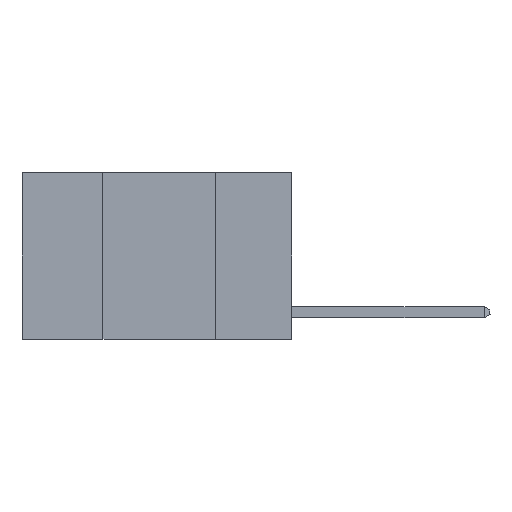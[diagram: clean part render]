
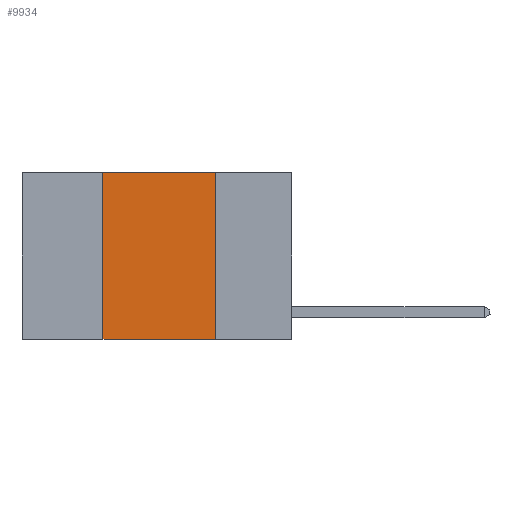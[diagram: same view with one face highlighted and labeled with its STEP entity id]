
A CAD part, left-side view. The second image highlights one B-rep face of the part: STEP entity #9934.
In plain terms, the highlighted planar face has unit normal (-1, 0, 0).
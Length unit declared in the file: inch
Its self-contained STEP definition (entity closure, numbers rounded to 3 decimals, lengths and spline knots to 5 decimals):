
#4 = VERTEX_POINT ( 'NONE', #1848 ) ;
#546 = CARTESIAN_POINT ( 'NONE',  ( 0., 0.6, 0. ) ) ;
#758 = PLANE ( 'NONE',  #8987 ) ;
#1290 = DIRECTION ( 'NONE',  ( 0., -1., 0. ) ) ;
#1499 = DIRECTION ( 'NONE',  ( 0., 0., -1. ) ) ;
#1561 = CARTESIAN_POINT ( 'NONE',  ( 0., 0.17, -0.37 ) ) ;
#1847 = CARTESIAN_POINT ( 'NONE',  ( 0., 0.42, 0. ) ) ;
#1848 = CARTESIAN_POINT ( 'NONE',  ( 0., 0.42, -0.37 ) ) ;
#2092 = ORIENTED_EDGE ( 'NONE', *, *, #6018, .F. ) ;
#2715 = EDGE_CURVE ( 'NONE', #12588, #7052, #3069, .T. ) ;
#3069 = LINE ( 'NONE', #5979, #9298 ) ;
#3140 = DIRECTION ( 'NONE',  ( 0., 0., -1. ) ) ;
#3213 = LINE ( 'NONE', #10354, #8958 ) ;
#3271 = VERTEX_POINT ( 'NONE', #7011 ) ;
#3482 = VECTOR ( 'NONE', #6341, 39.37008 ) ;
#4774 = DIRECTION ( 'NONE',  ( 0., 0., 1. ) ) ;
#5296 = ORIENTED_EDGE ( 'NONE', *, *, #9792, .F. ) ;
#5979 = CARTESIAN_POINT ( 'NONE',  ( 0., 0.17, 0. ) ) ;
#5982 = VECTOR ( 'NONE', #4774, 39.37008 ) ;
#6018 = EDGE_CURVE ( 'NONE', #4, #3271, #9801, .T. ) ;
#6341 = DIRECTION ( 'NONE',  ( 0., -1., 0. ) ) ;
#6407 = EDGE_LOOP ( 'NONE', ( #6683, #5296, #2092, #9601 ) ) ;
#6660 = FACE_OUTER_BOUND ( 'NONE', #6407, .T. ) ;
#6683 = ORIENTED_EDGE ( 'NONE', *, *, #2715, .F. ) ;
#6940 = CARTESIAN_POINT ( 'NONE',  ( 0., 0.17, 0. ) ) ;
#7011 = CARTESIAN_POINT ( 'NONE',  ( 0., 0.42, 0. ) ) ;
#7052 = VERTEX_POINT ( 'NONE', #1561 ) ;
#8502 = EDGE_CURVE ( 'NONE', #4, #7052, #3213, .T. ) ;
#8958 = VECTOR ( 'NONE', #1290, 39.37008 ) ;
#8987 = AXIS2_PLACEMENT_3D ( 'NONE', #546, #10625, #1499 ) ;
#9261 = LINE ( 'NONE', #9452, #3482 ) ;
#9298 = VECTOR ( 'NONE', #3140, 39.37008 ) ;
#9452 = CARTESIAN_POINT ( 'NONE',  ( 0., 0.6, 0. ) ) ;
#9601 = ORIENTED_EDGE ( 'NONE', *, *, #8502, .T. ) ;
#9792 = EDGE_CURVE ( 'NONE', #3271, #12588, #9261, .T. ) ;
#9801 = LINE ( 'NONE', #1847, #5982 ) ;
#9934 = ADVANCED_FACE ( 'NONE', ( #6660 ), #758, .F. ) ;
#10354 = CARTESIAN_POINT ( 'NONE',  ( 0., 0.6, -0.37 ) ) ;
#10625 = DIRECTION ( 'NONE',  ( 1., 0., 0. ) ) ;
#12588 = VERTEX_POINT ( 'NONE', #6940 ) ;
